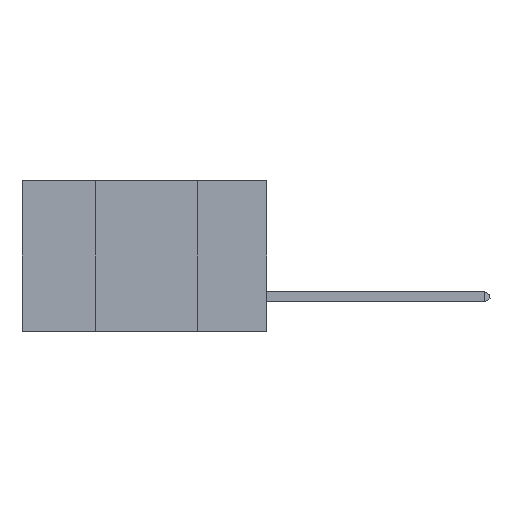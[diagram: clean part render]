
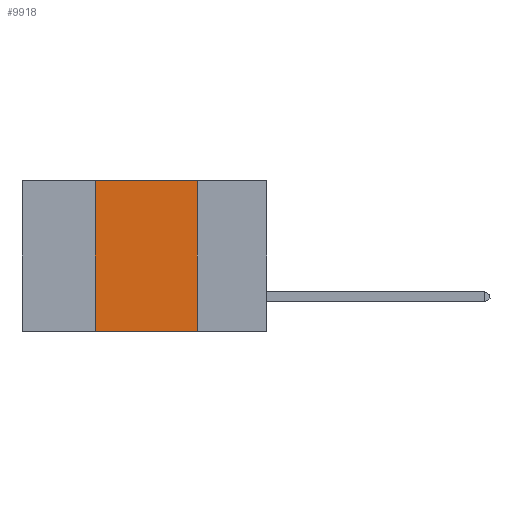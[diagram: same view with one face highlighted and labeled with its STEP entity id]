
A CAD part, left-side view. The second image highlights one B-rep face of the part: STEP entity #9918.
In plain terms, the highlighted planar face has unit normal (-1, 0, 0).
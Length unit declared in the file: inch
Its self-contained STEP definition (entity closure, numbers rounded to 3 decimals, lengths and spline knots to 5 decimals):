
#1007 = VECTOR ( 'NONE', #1969, 39.37008 ) ;
#1969 = DIRECTION ( 'NONE',  ( 0., 0., -1. ) ) ;
#3458 = ORIENTED_EDGE ( 'NONE', *, *, #31280, .T. ) ;
#4515 = CARTESIAN_POINT ( 'NONE',  ( 0., 0.17, -0.37 ) ) ;
#5209 = LINE ( 'NONE', #24558, #36256 ) ;
#5937 = CARTESIAN_POINT ( 'NONE',  ( 0., 0.17, 0. ) ) ;
#6079 = CARTESIAN_POINT ( 'NONE',  ( 0., 0.42, 0. ) ) ;
#7062 = CARTESIAN_POINT ( 'NONE',  ( 0., 0.6, 0. ) ) ;
#7104 = DIRECTION ( 'NONE',  ( 0., -1., 0. ) ) ;
#7902 = LINE ( 'NONE', #31123, #1007 ) ;
#9330 = CARTESIAN_POINT ( 'NONE',  ( 0., 0.6, -0.37 ) ) ;
#9918 = ADVANCED_FACE ( 'NONE', ( #36359 ), #21568, .F. ) ;
#9971 = DIRECTION ( 'NONE',  ( 0., 0., -1. ) ) ;
#10654 = VERTEX_POINT ( 'NONE', #4515 ) ;
#11226 = EDGE_CURVE ( 'NONE', #33940, #36608, #5209, .T. ) ;
#11497 = ORIENTED_EDGE ( 'NONE', *, *, #36390, .F. ) ;
#12228 = DIRECTION ( 'NONE',  ( 0., -1., 0. ) ) ;
#12858 = EDGE_CURVE ( 'NONE', #15602, #33940, #16010, .T. ) ;
#14819 = CARTESIAN_POINT ( 'NONE',  ( 0., 0.42, -0.37 ) ) ;
#15602 = VERTEX_POINT ( 'NONE', #14819 ) ;
#15674 = ORIENTED_EDGE ( 'NONE', *, *, #12858, .F. ) ;
#16010 = LINE ( 'NONE', #6079, #37554 ) ;
#20663 = DIRECTION ( 'NONE',  ( 0., 0., 1. ) ) ;
#21568 = PLANE ( 'NONE',  #28923 ) ;
#24558 = CARTESIAN_POINT ( 'NONE',  ( 0., 0.6, 0. ) ) ;
#25076 = CARTESIAN_POINT ( 'NONE',  ( 0., 0.42, 0. ) ) ;
#27509 = DIRECTION ( 'NONE',  ( 1., 0., 0. ) ) ;
#28923 = AXIS2_PLACEMENT_3D ( 'NONE', #7062, #27509, #9971 ) ;
#31123 = CARTESIAN_POINT ( 'NONE',  ( 0., 0.17, 0. ) ) ;
#31280 = EDGE_CURVE ( 'NONE', #15602, #10654, #36555, .T. ) ;
#33940 = VERTEX_POINT ( 'NONE', #25076 ) ;
#34734 = VECTOR ( 'NONE', #12228, 39.37008 ) ;
#34998 = ORIENTED_EDGE ( 'NONE', *, *, #11226, .F. ) ;
#36256 = VECTOR ( 'NONE', #7104, 39.37008 ) ;
#36359 = FACE_OUTER_BOUND ( 'NONE', #36642, .T. ) ;
#36390 = EDGE_CURVE ( 'NONE', #36608, #10654, #7902, .T. ) ;
#36555 = LINE ( 'NONE', #9330, #34734 ) ;
#36608 = VERTEX_POINT ( 'NONE', #5937 ) ;
#36642 = EDGE_LOOP ( 'NONE', ( #11497, #34998, #15674, #3458 ) ) ;
#37554 = VECTOR ( 'NONE', #20663, 39.37008 ) ;
